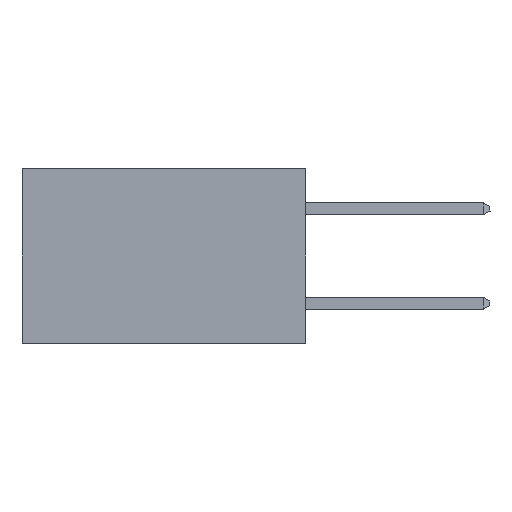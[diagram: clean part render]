
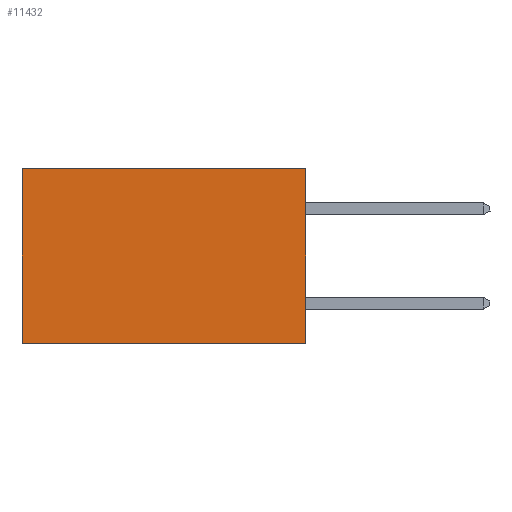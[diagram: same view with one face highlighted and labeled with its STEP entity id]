
A CAD part, left-side view. The second image highlights one B-rep face of the part: STEP entity #11432.
In plain terms, the highlighted planar face has unit normal (-1, 0, 0).
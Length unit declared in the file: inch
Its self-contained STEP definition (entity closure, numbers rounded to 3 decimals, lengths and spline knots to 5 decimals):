
#131 = EDGE_CURVE ( 'NONE', #10397, #5874, #11033, .T. ) ;
#172 = LINE ( 'NONE', #2053, #3426 ) ;
#440 = DIRECTION ( 'NONE',  ( 1., 0., 0. ) ) ;
#470 = ORIENTED_EDGE ( 'NONE', *, *, #7112, .T. ) ;
#645 = LINE ( 'NONE', #7118, #8327 ) ;
#1426 = CARTESIAN_POINT ( 'NONE',  ( 0.298, 0., 0. ) ) ;
#2053 = CARTESIAN_POINT ( 'NONE',  ( 0.298, 0.6, 0. ) ) ;
#2085 = ORIENTED_EDGE ( 'NONE', *, *, #8177, .T. ) ;
#2930 = FACE_OUTER_BOUND ( 'NONE', #6465, .T. ) ;
#3157 = VECTOR ( 'NONE', #3919, 39.37008 ) ;
#3293 = DIRECTION ( 'NONE',  ( 0., 0., -1. ) ) ;
#3426 = VECTOR ( 'NONE', #4051, 39.37008 ) ;
#3678 = AXIS2_PLACEMENT_3D ( 'NONE', #6112, #440, #3293 ) ;
#3919 = DIRECTION ( 'NONE',  ( 0., 1., 0. ) ) ;
#4051 = DIRECTION ( 'NONE',  ( 0., 0., -1. ) ) ;
#4262 = DIRECTION ( 'NONE',  ( 0., 1., 0. ) ) ;
#4859 = VECTOR ( 'NONE', #7276, 39.37008 ) ;
#5460 = LINE ( 'NONE', #10190, #4859 ) ;
#5874 = VERTEX_POINT ( 'NONE', #12108 ) ;
#6112 = CARTESIAN_POINT ( 'NONE',  ( 0.298, 0., 0. ) ) ;
#6439 = CARTESIAN_POINT ( 'NONE',  ( 0.298, 0.6, 0. ) ) ;
#6465 = EDGE_LOOP ( 'NONE', ( #2085, #10918, #9436, #470 ) ) ;
#6754 = VERTEX_POINT ( 'NONE', #6439 ) ;
#7112 = EDGE_CURVE ( 'NONE', #12111, #6754, #645, .T. ) ;
#7118 = CARTESIAN_POINT ( 'NONE',  ( 0.298, 0., 0. ) ) ;
#7147 = PLANE ( 'NONE',  #3678 ) ;
#7276 = DIRECTION ( 'NONE',  ( 0., 0., -1. ) ) ;
#8177 = EDGE_CURVE ( 'NONE', #6754, #5874, #172, .T. ) ;
#8327 = VECTOR ( 'NONE', #4262, 39.37008 ) ;
#9436 = ORIENTED_EDGE ( 'NONE', *, *, #11590, .F. ) ;
#9695 = CARTESIAN_POINT ( 'NONE',  ( 0.298, 0., -0.37 ) ) ;
#10190 = CARTESIAN_POINT ( 'NONE',  ( 0.298, 0., 0. ) ) ;
#10213 = CARTESIAN_POINT ( 'NONE',  ( 0.298, 0., -0.37 ) ) ;
#10397 = VERTEX_POINT ( 'NONE', #10213 ) ;
#10918 = ORIENTED_EDGE ( 'NONE', *, *, #131, .F. ) ;
#11033 = LINE ( 'NONE', #9695, #3157 ) ;
#11432 = ADVANCED_FACE ( 'NONE', ( #2930 ), #7147, .F. ) ;
#11590 = EDGE_CURVE ( 'NONE', #12111, #10397, #5460, .T. ) ;
#12108 = CARTESIAN_POINT ( 'NONE',  ( 0.298, 0.6, -0.37 ) ) ;
#12111 = VERTEX_POINT ( 'NONE', #1426 ) ;
